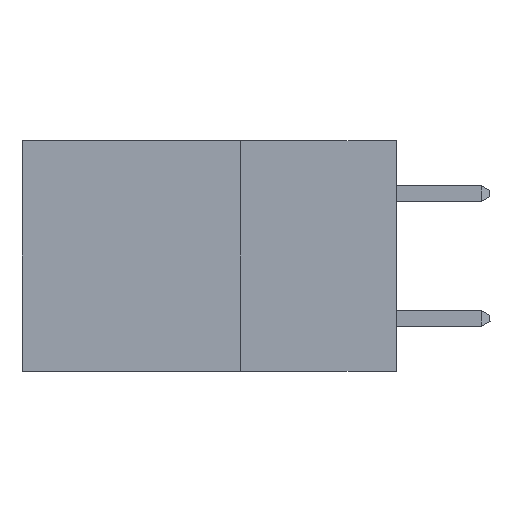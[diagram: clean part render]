
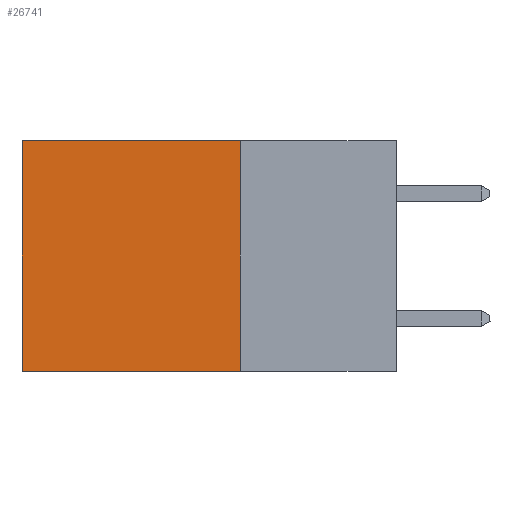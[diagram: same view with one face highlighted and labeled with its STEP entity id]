
A CAD part, left-side view. The second image highlights one B-rep face of the part: STEP entity #26741.
In plain terms, the highlighted planar face has unit normal (-1, 0, 0).
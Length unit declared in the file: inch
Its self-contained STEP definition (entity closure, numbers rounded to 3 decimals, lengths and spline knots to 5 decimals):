
#897 = VERTEX_POINT ( 'NONE', #3959 ) ;
#1102 = PLANE ( 'NONE',  #28863 ) ;
#1504 = EDGE_LOOP ( 'NONE', ( #8953, #22565, #4219, #5784 ) ) ;
#3028 = CARTESIAN_POINT ( 'NONE',  ( 0.298, 0.25, 0. ) ) ;
#3959 = CARTESIAN_POINT ( 'NONE',  ( 0.298, 0.25, -0.37 ) ) ;
#4219 = ORIENTED_EDGE ( 'NONE', *, *, #16573, .F. ) ;
#4351 = VERTEX_POINT ( 'NONE', #13009 ) ;
#4997 = EDGE_CURVE ( 'NONE', #10940, #21799, #5247, .T. ) ;
#5247 = LINE ( 'NONE', #25285, #23376 ) ;
#5495 = DIRECTION ( 'NONE',  ( 0., 1., 0. ) ) ;
#5784 = ORIENTED_EDGE ( 'NONE', *, *, #10017, .T. ) ;
#6061 = DIRECTION ( 'NONE',  ( 1., 0., 0. ) ) ;
#6541 = VECTOR ( 'NONE', #17705, 39.37008 ) ;
#8431 = DIRECTION ( 'NONE',  ( 0., 1., 0. ) ) ;
#8953 = ORIENTED_EDGE ( 'NONE', *, *, #4997, .T. ) ;
#10017 = EDGE_CURVE ( 'NONE', #4351, #10940, #20812, .T. ) ;
#10940 = VERTEX_POINT ( 'NONE', #11692 ) ;
#11692 = CARTESIAN_POINT ( 'NONE',  ( 0.298, 0.6, 0. ) ) ;
#13009 = CARTESIAN_POINT ( 'NONE',  ( 0.298, 0.25, 0. ) ) ;
#13122 = LINE ( 'NONE', #22592, #6541 ) ;
#13529 = VECTOR ( 'NONE', #5495, 39.37008 ) ;
#16573 = EDGE_CURVE ( 'NONE', #4351, #897, #13122, .T. ) ;
#17252 = VECTOR ( 'NONE', #8431, 39.37008 ) ;
#17705 = DIRECTION ( 'NONE',  ( 0., 0., -1. ) ) ;
#19232 = FACE_OUTER_BOUND ( 'NONE', #1504, .T. ) ;
#20460 = CARTESIAN_POINT ( 'NONE',  ( 0.298, 0.6, -0.37 ) ) ;
#20797 = CARTESIAN_POINT ( 'NONE',  ( 0.298, 0.25, 0. ) ) ;
#20812 = LINE ( 'NONE', #3028, #13529 ) ;
#21799 = VERTEX_POINT ( 'NONE', #20460 ) ;
#22565 = ORIENTED_EDGE ( 'NONE', *, *, #22574, .F. ) ;
#22574 = EDGE_CURVE ( 'NONE', #897, #21799, #30458, .T. ) ;
#22592 = CARTESIAN_POINT ( 'NONE',  ( 0.298, 0.25, 0. ) ) ;
#23306 = DIRECTION ( 'NONE',  ( 0., 0., -1. ) ) ;
#23376 = VECTOR ( 'NONE', #25396, 39.37008 ) ;
#25285 = CARTESIAN_POINT ( 'NONE',  ( 0.298, 0.6, 0. ) ) ;
#25396 = DIRECTION ( 'NONE',  ( 0., 0., -1. ) ) ;
#25722 = CARTESIAN_POINT ( 'NONE',  ( 0.298, 0.25, -0.37 ) ) ;
#26741 = ADVANCED_FACE ( 'NONE', ( #19232 ), #1102, .F. ) ;
#28863 = AXIS2_PLACEMENT_3D ( 'NONE', #20797, #6061, #23306 ) ;
#30458 = LINE ( 'NONE', #25722, #17252 ) ;
